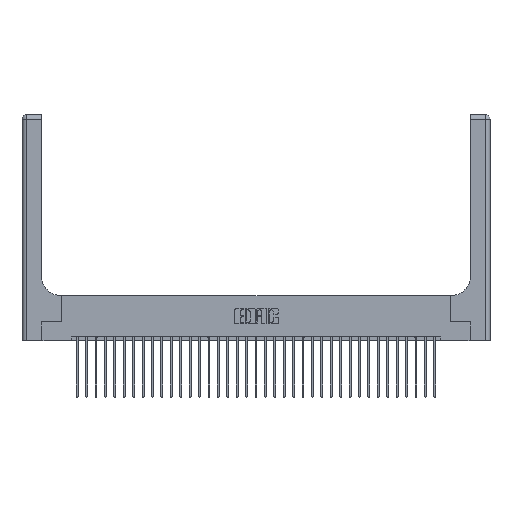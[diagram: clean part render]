
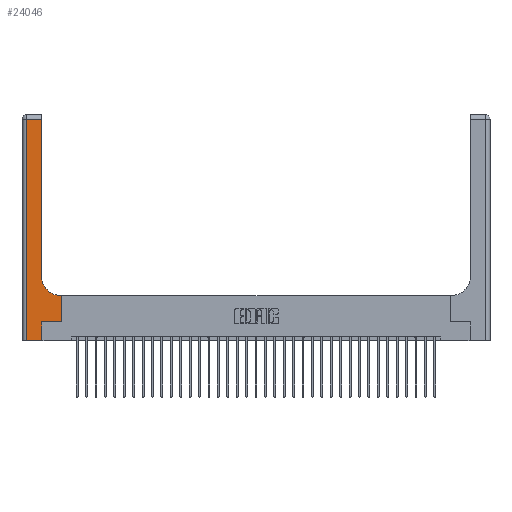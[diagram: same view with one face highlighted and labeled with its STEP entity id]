
A CAD part, top view. The second image highlights one B-rep face of the part: STEP entity #24046.
In plain terms, the highlighted planar face has unit normal (0, 0, 1).
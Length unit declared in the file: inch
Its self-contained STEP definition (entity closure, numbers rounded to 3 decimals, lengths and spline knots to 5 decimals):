
#200 = LINE ( 'NONE', #8277, #11114 ) ;
#421 = VERTEX_POINT ( 'NONE', #27889 ) ;
#850 = CARTESIAN_POINT ( 'NONE',  ( 0.26, 0.6, 0.37 ) ) ;
#966 = EDGE_CURVE ( 'NONE', #26807, #22726, #15951, .T. ) ;
#1298 = DIRECTION ( 'NONE',  ( 0., 1., 0. ) ) ;
#2137 = ORIENTED_EDGE ( 'NONE', *, *, #13906, .T. ) ;
#2908 = PLANE ( 'NONE',  #9421 ) ;
#3025 = ORIENTED_EDGE ( 'NONE', *, *, #30345, .T. ) ;
#3304 = VECTOR ( 'NONE', #8954, 39.37008 ) ;
#3487 = CARTESIAN_POINT ( 'NONE',  ( 0.26, 3., 0.37 ) ) ;
#4922 = CARTESIAN_POINT ( 'NONE',  ( 0.528, 0.25, 0.37 ) ) ;
#5405 = DIRECTION ( 'NONE',  ( 0., 0., -1. ) ) ;
#5438 = ORIENTED_EDGE ( 'NONE', *, *, #15025, .T. ) ;
#5443 = VECTOR ( 'NONE', #14660, 39.37008 ) ;
#6732 = DIRECTION ( 'NONE',  ( 1., 0., 0. ) ) ;
#7528 = CARTESIAN_POINT ( 'NONE',  ( 0., 2.94, 0.37 ) ) ;
#7976 = VERTEX_POINT ( 'NONE', #26070 ) ;
#7985 = VECTOR ( 'NONE', #1298, 39.37008 ) ;
#8040 = ORIENTED_EDGE ( 'NONE', *, *, #29101, .T. ) ;
#8109 = CARTESIAN_POINT ( 'NONE',  ( 0.265, 0., 0.37 ) ) ;
#8277 = CARTESIAN_POINT ( 'NONE',  ( 0.06, 3., 0.37 ) ) ;
#8934 = EDGE_CURVE ( 'NONE', #28631, #24468, #25387, .T. ) ;
#8954 = DIRECTION ( 'NONE',  ( 1., 0., 0. ) ) ;
#9362 = CARTESIAN_POINT ( 'NONE',  ( 0.528, 0.6, 0.37 ) ) ;
#9421 = AXIS2_PLACEMENT_3D ( 'NONE', #17382, #5405, #29233 ) ;
#9817 = CIRCLE ( 'NONE', #11859, 0.25 ) ;
#10894 = CARTESIAN_POINT ( 'NONE',  ( 0.26, 0.85, 0.37 ) ) ;
#11114 = VECTOR ( 'NONE', #15335, 39.37008 ) ;
#11276 = EDGE_CURVE ( 'NONE', #19469, #20656, #15134, .T. ) ;
#11453 = ORIENTED_EDGE ( 'NONE', *, *, #11276, .T. ) ;
#11859 = AXIS2_PLACEMENT_3D ( 'NONE', #28638, #14272, #6732 ) ;
#12010 = EDGE_CURVE ( 'NONE', #22726, #19469, #9817, .T. ) ;
#12523 = LINE ( 'NONE', #7528, #29067 ) ;
#13715 = CARTESIAN_POINT ( 'NONE',  ( 0.528, 0.25, 0.37 ) ) ;
#13767 = ORIENTED_EDGE ( 'NONE', *, *, #12010, .T. ) ;
#13906 = EDGE_CURVE ( 'NONE', #24468, #25797, #16834, .T. ) ;
#14272 = DIRECTION ( 'NONE',  ( 0., 0., -1. ) ) ;
#14296 = CARTESIAN_POINT ( 'NONE',  ( 0., 0., 0.37 ) ) ;
#14660 = DIRECTION ( 'NONE',  ( 0., 1., 0. ) ) ;
#15025 = EDGE_CURVE ( 'NONE', #7976, #421, #200, .T. ) ;
#15134 = LINE ( 'NONE', #3487, #7985 ) ;
#15335 = DIRECTION ( 'NONE',  ( 0., -1., 0. ) ) ;
#15951 = LINE ( 'NONE', #850, #25711 ) ;
#16102 = LINE ( 'NONE', #13715, #17195 ) ;
#16834 = LINE ( 'NONE', #28181, #3304 ) ;
#17195 = VECTOR ( 'NONE', #18510, 39.37008 ) ;
#17382 = CARTESIAN_POINT ( 'NONE',  ( 0., 3., 0.37 ) ) ;
#17962 = EDGE_CURVE ( 'NONE', #25797, #26807, #16102, .T. ) ;
#18463 = CARTESIAN_POINT ( 'NONE',  ( 0.26, 2.94, 0.37 ) ) ;
#18510 = DIRECTION ( 'NONE',  ( 0., 1., 0. ) ) ;
#19233 = FACE_OUTER_BOUND ( 'NONE', #22898, .T. ) ;
#19469 = VERTEX_POINT ( 'NONE', #10894 ) ;
#20053 = VECTOR ( 'NONE', #26455, 39.37008 ) ;
#20178 = DIRECTION ( 'NONE',  ( -1., 0., 0. ) ) ;
#20656 = VERTEX_POINT ( 'NONE', #18463 ) ;
#21180 = LINE ( 'NONE', #14296, #20053 ) ;
#21293 = CARTESIAN_POINT ( 'NONE',  ( 0.51, 0.6, 0.37 ) ) ;
#21731 = CARTESIAN_POINT ( 'NONE',  ( 0.265, 0., 0.37 ) ) ;
#22506 = DIRECTION ( 'NONE',  ( -1., 0., 0. ) ) ;
#22726 = VERTEX_POINT ( 'NONE', #21293 ) ;
#22898 = EDGE_LOOP ( 'NONE', ( #11453, #8040, #5438, #3025, #30049, #2137, #27398, #29724, #13767 ) ) ;
#24046 = ADVANCED_FACE ( 'NONE', ( #19233 ), #2908, .F. ) ;
#24468 = VERTEX_POINT ( 'NONE', #26581 ) ;
#25387 = LINE ( 'NONE', #21731, #5443 ) ;
#25711 = VECTOR ( 'NONE', #22506, 39.37008 ) ;
#25797 = VERTEX_POINT ( 'NONE', #4922 ) ;
#26070 = CARTESIAN_POINT ( 'NONE',  ( 0.06, 2.94, 0.37 ) ) ;
#26455 = DIRECTION ( 'NONE',  ( 1., 0., 0. ) ) ;
#26581 = CARTESIAN_POINT ( 'NONE',  ( 0.265, 0.25, 0.37 ) ) ;
#26807 = VERTEX_POINT ( 'NONE', #9362 ) ;
#27398 = ORIENTED_EDGE ( 'NONE', *, *, #17962, .T. ) ;
#27889 = CARTESIAN_POINT ( 'NONE',  ( 0.06, 0., 0.37 ) ) ;
#28181 = CARTESIAN_POINT ( 'NONE',  ( 0.265, 0.25, 0.37 ) ) ;
#28631 = VERTEX_POINT ( 'NONE', #8109 ) ;
#28638 = CARTESIAN_POINT ( 'NONE',  ( 0.51, 0.85, 0.37 ) ) ;
#29067 = VECTOR ( 'NONE', #20178, 39.37008 ) ;
#29101 = EDGE_CURVE ( 'NONE', #20656, #7976, #12523, .T. ) ;
#29233 = DIRECTION ( 'NONE',  ( -1., 0., 0. ) ) ;
#29724 = ORIENTED_EDGE ( 'NONE', *, *, #966, .T. ) ;
#30049 = ORIENTED_EDGE ( 'NONE', *, *, #8934, .T. ) ;
#30345 = EDGE_CURVE ( 'NONE', #421, #28631, #21180, .T. ) ;
